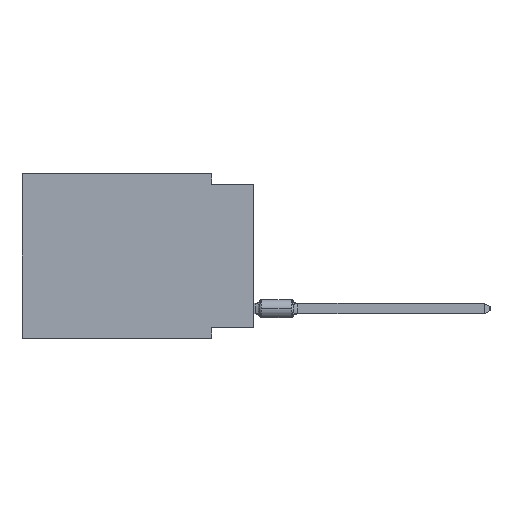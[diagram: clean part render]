
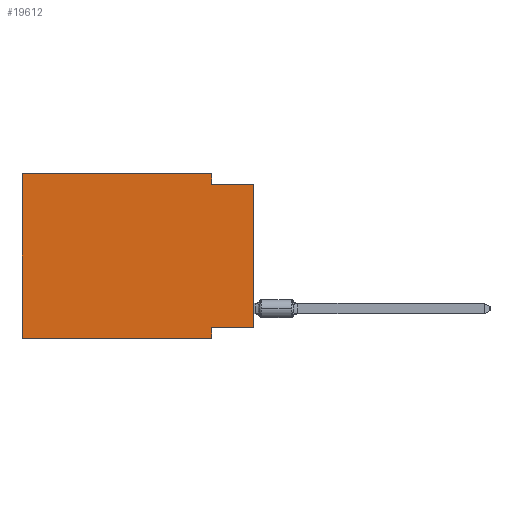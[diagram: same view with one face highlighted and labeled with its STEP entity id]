
A CAD part, left-side view. The second image highlights one B-rep face of the part: STEP entity #19612.
In plain terms, the highlighted planar face has unit normal (-1, 0, 0).
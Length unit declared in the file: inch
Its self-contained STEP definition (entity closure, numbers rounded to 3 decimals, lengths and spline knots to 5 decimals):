
#380 = CARTESIAN_POINT ( 'NONE',  ( 0., 0.1, -0.365 ) ) ;
#497 = LINE ( 'NONE', #18827, #13092 ) ;
#552 = CARTESIAN_POINT ( 'NONE',  ( 0., 0.55, -0.39 ) ) ;
#704 = DIRECTION ( 'NONE',  ( 0., 0., 1. ) ) ;
#961 = CARTESIAN_POINT ( 'NONE',  ( 0., 0., -0.025 ) ) ;
#1428 = CARTESIAN_POINT ( 'NONE',  ( 0., 0.1, -0.39 ) ) ;
#1868 = CARTESIAN_POINT ( 'NONE',  ( 0., 0., -0.025 ) ) ;
#2285 = EDGE_CURVE ( 'NONE', #23881, #18521, #10896, .T. ) ;
#3595 = EDGE_CURVE ( 'NONE', #20329, #29237, #497, .T. ) ;
#3653 = VECTOR ( 'NONE', #27094, 39.37008 ) ;
#4672 = ORIENTED_EDGE ( 'NONE', *, *, #28889, .F. ) ;
#5587 = CARTESIAN_POINT ( 'NONE',  ( 0., 0.55, 0. ) ) ;
#5599 = CARTESIAN_POINT ( 'NONE',  ( 0., 0.1, 0. ) ) ;
#5689 = CARTESIAN_POINT ( 'NONE',  ( 0., 0., 0. ) ) ;
#5909 = ORIENTED_EDGE ( 'NONE', *, *, #21666, .F. ) ;
#6175 = DIRECTION ( 'NONE',  ( 0., -1., 0. ) ) ;
#6583 = VERTEX_POINT ( 'NONE', #1428 ) ;
#7668 = FACE_OUTER_BOUND ( 'NONE', #11922, .T. ) ;
#8221 = ORIENTED_EDGE ( 'NONE', *, *, #18534, .T. ) ;
#8462 = CARTESIAN_POINT ( 'NONE',  ( 0., 0.1, -0.025 ) ) ;
#8889 = LINE ( 'NONE', #22918, #13071 ) ;
#8987 = CARTESIAN_POINT ( 'NONE',  ( 0., 0.55, 0. ) ) ;
#9880 = VECTOR ( 'NONE', #13091, 39.37008 ) ;
#10737 = EDGE_CURVE ( 'NONE', #26629, #6583, #29190, .T. ) ;
#10896 = LINE ( 'NONE', #1868, #19715 ) ;
#11511 = CARTESIAN_POINT ( 'NONE',  ( 0., 0.55, 0. ) ) ;
#11650 = LINE ( 'NONE', #11511, #21535 ) ;
#11922 = EDGE_LOOP ( 'NONE', ( #8221, #25223, #15261, #5909, #17818, #13400, #4672, #25360 ) ) ;
#12108 = DIRECTION ( 'NONE',  ( 1., 0., 0. ) ) ;
#12962 = DIRECTION ( 'NONE',  ( 0., -1., 0. ) ) ;
#13071 = VECTOR ( 'NONE', #20707, 39.37008 ) ;
#13091 = DIRECTION ( 'NONE',  ( 0., -1., 0. ) ) ;
#13092 = VECTOR ( 'NONE', #18535, 39.37008 ) ;
#13400 = ORIENTED_EDGE ( 'NONE', *, *, #10737, .T. ) ;
#13697 = EDGE_CURVE ( 'NONE', #20927, #23881, #27380, .T. ) ;
#14225 = CARTESIAN_POINT ( 'NONE',  ( 0., 0.1, 0. ) ) ;
#14701 = DIRECTION ( 'NONE',  ( 0., 0., 1. ) ) ;
#15261 = ORIENTED_EDGE ( 'NONE', *, *, #13697, .F. ) ;
#15874 = VECTOR ( 'NONE', #12962, 39.37008 ) ;
#16690 = CARTESIAN_POINT ( 'NONE',  ( 0., 0.55, 0. ) ) ;
#17818 = ORIENTED_EDGE ( 'NONE', *, *, #26507, .F. ) ;
#17941 = CARTESIAN_POINT ( 'NONE',  ( 0., 0.55, -0.39 ) ) ;
#18521 = VERTEX_POINT ( 'NONE', #961 ) ;
#18534 = EDGE_CURVE ( 'NONE', #20329, #18521, #25951, .T. ) ;
#18535 = DIRECTION ( 'NONE',  ( 0., 1., 0. ) ) ;
#18745 = PLANE ( 'NONE',  #21832 ) ;
#18827 = CARTESIAN_POINT ( 'NONE',  ( 0., 0., -0.365 ) ) ;
#19612 = ADVANCED_FACE ( 'NONE', ( #7668 ), #18745, .F. ) ;
#19715 = VECTOR ( 'NONE', #6175, 39.37008 ) ;
#20329 = VERTEX_POINT ( 'NONE', #22921 ) ;
#20707 = DIRECTION ( 'NONE',  ( 0., 0., -1. ) ) ;
#20927 = VERTEX_POINT ( 'NONE', #5599 ) ;
#21123 = DIRECTION ( 'NONE',  ( 0., 0., -1. ) ) ;
#21535 = VECTOR ( 'NONE', #704, 39.37008 ) ;
#21666 = EDGE_CURVE ( 'NONE', #26354, #20927, #24035, .T. ) ;
#21786 = VECTOR ( 'NONE', #14701, 39.37008 ) ;
#21832 = AXIS2_PLACEMENT_3D ( 'NONE', #16690, #12108, #21123 ) ;
#22918 = CARTESIAN_POINT ( 'NONE',  ( 0., 0.1, -0.39 ) ) ;
#22921 = CARTESIAN_POINT ( 'NONE',  ( 0., 0., -0.365 ) ) ;
#23881 = VERTEX_POINT ( 'NONE', #8462 ) ;
#24035 = LINE ( 'NONE', #5587, #15874 ) ;
#25223 = ORIENTED_EDGE ( 'NONE', *, *, #2285, .F. ) ;
#25360 = ORIENTED_EDGE ( 'NONE', *, *, #3595, .F. ) ;
#25951 = LINE ( 'NONE', #5689, #21786 ) ;
#26354 = VERTEX_POINT ( 'NONE', #8987 ) ;
#26507 = EDGE_CURVE ( 'NONE', #26629, #26354, #11650, .T. ) ;
#26629 = VERTEX_POINT ( 'NONE', #552 ) ;
#27094 = DIRECTION ( 'NONE',  ( 0., 0., -1. ) ) ;
#27380 = LINE ( 'NONE', #14225, #3653 ) ;
#28889 = EDGE_CURVE ( 'NONE', #29237, #6583, #8889, .T. ) ;
#29190 = LINE ( 'NONE', #17941, #9880 ) ;
#29237 = VERTEX_POINT ( 'NONE', #380 ) ;
